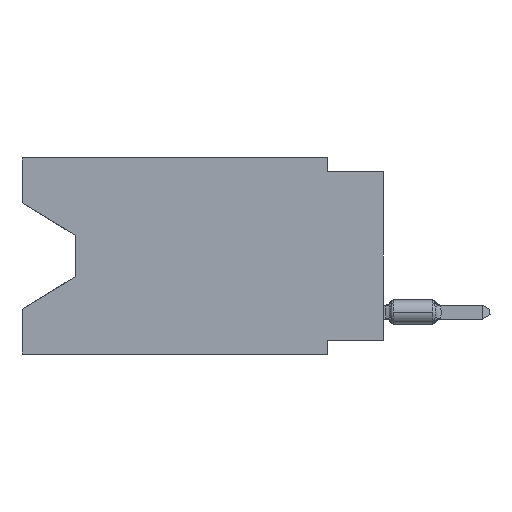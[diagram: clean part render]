
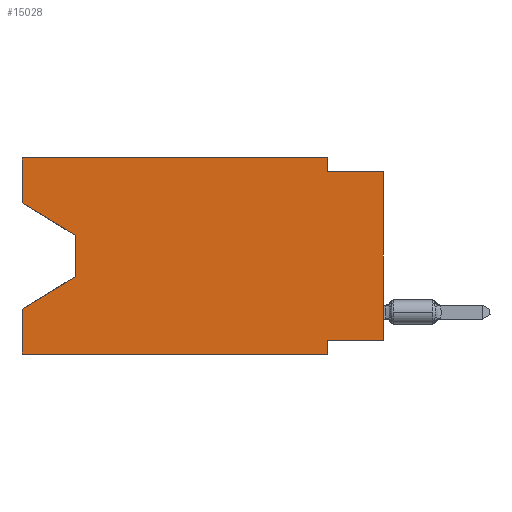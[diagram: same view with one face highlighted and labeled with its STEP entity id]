
A CAD part, left-side view. The second image highlights one B-rep face of the part: STEP entity #15028.
In plain terms, the highlighted planar face has unit normal (-1, 0, 0).
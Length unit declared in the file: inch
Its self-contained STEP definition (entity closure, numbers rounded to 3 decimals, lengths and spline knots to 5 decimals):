
#46 = CARTESIAN_POINT ( 'NONE',  ( 0., 0.645, 0. ) ) ;
#237 = DIRECTION ( 'NONE',  ( 1., 0., 0. ) ) ;
#358 = EDGE_CURVE ( 'NONE', #9131, #15385, #25712, .T. ) ;
#706 = CARTESIAN_POINT ( 'NONE',  ( 0., 0.645, 0. ) ) ;
#745 = VECTOR ( 'NONE', #42274, 39.37008 ) ;
#879 = CARTESIAN_POINT ( 'NONE',  ( 0., 0., -0.025 ) ) ;
#1329 = EDGE_LOOP ( 'NONE', ( #43893, #31554, #24257, #16277, #18783, #42385, #1953, #32774, #33896, #38609, #2377, #43063 ) ) ;
#1415 = DIRECTION ( 'NONE',  ( 0., -0.855, -0.519 ) ) ;
#1826 = VECTOR ( 'NONE', #4536, 39.37008 ) ;
#1953 = ORIENTED_EDGE ( 'NONE', *, *, #17842, .F. ) ;
#2377 = ORIENTED_EDGE ( 'NONE', *, *, #33016, .F. ) ;
#3323 = DIRECTION ( 'NONE',  ( 0., 0., -1. ) ) ;
#3434 = VERTEX_POINT ( 'NONE', #34422 ) ;
#3835 = CARTESIAN_POINT ( 'NONE',  ( 0., 0.645, -0.26975 ) ) ;
#4311 = LINE ( 'NONE', #879, #1826 ) ;
#4511 = VERTEX_POINT ( 'NONE', #46 ) ;
#4536 = DIRECTION ( 'NONE',  ( 0., -1., 0. ) ) ;
#5310 = LINE ( 'NONE', #26547, #37855 ) ;
#5850 = CARTESIAN_POINT ( 'NONE',  ( 0., 0.1, 0. ) ) ;
#7268 = VECTOR ( 'NONE', #38664, 39.37008 ) ;
#7551 = PLANE ( 'NONE',  #43920 ) ;
#8759 = VECTOR ( 'NONE', #3323, 39.37008 ) ;
#9131 = VERTEX_POINT ( 'NONE', #44432 ) ;
#9416 = VECTOR ( 'NONE', #21466, 39.37008 ) ;
#10140 = CARTESIAN_POINT ( 'NONE',  ( 0., 0., -0.025 ) ) ;
#10227 = CARTESIAN_POINT ( 'NONE',  ( 0., 0.1, -0.35 ) ) ;
#11408 = CARTESIAN_POINT ( 'NONE',  ( 0., 0.645, -0.35 ) ) ;
#11585 = CARTESIAN_POINT ( 'NONE',  ( 0., 0.55, -0.212 ) ) ;
#12826 = EDGE_CURVE ( 'NONE', #31599, #22382, #44892, .T. ) ;
#13238 = CARTESIAN_POINT ( 'NONE',  ( 0., 0.55, -0.138 ) ) ;
#14643 = LINE ( 'NONE', #706, #745 ) ;
#14780 = LINE ( 'NONE', #18657, #34609 ) ;
#14848 = CARTESIAN_POINT ( 'NONE',  ( 0., 0.645, 0. ) ) ;
#15028 = ADVANCED_FACE ( 'NONE', ( #18263 ), #7551, .F. ) ;
#15347 = VECTOR ( 'NONE', #32556, 39.37008 ) ;
#15385 = VERTEX_POINT ( 'NONE', #3835 ) ;
#16121 = DIRECTION ( 'NONE',  ( 0., 0., -1. ) ) ;
#16277 = ORIENTED_EDGE ( 'NONE', *, *, #358, .F. ) ;
#17458 = EDGE_CURVE ( 'NONE', #3434, #15385, #39215, .T. ) ;
#17842 = EDGE_CURVE ( 'NONE', #37685, #31599, #29112, .T. ) ;
#18263 = FACE_OUTER_BOUND ( 'NONE', #1329, .T. ) ;
#18418 = CARTESIAN_POINT ( 'NONE',  ( 0., 0.1, -0.325 ) ) ;
#18427 = DIRECTION ( 'NONE',  ( 0., -1., 0. ) ) ;
#18623 = CARTESIAN_POINT ( 'NONE',  ( 0., 0.645, 0. ) ) ;
#18657 = CARTESIAN_POINT ( 'NONE',  ( 0., 0.645, 0. ) ) ;
#18783 = ORIENTED_EDGE ( 'NONE', *, *, #40197, .T. ) ;
#19572 = CARTESIAN_POINT ( 'NONE',  ( 0., 0., 0. ) ) ;
#20453 = CARTESIAN_POINT ( 'NONE',  ( 0., 0.1, -0.35 ) ) ;
#21118 = VECTOR ( 'NONE', #39686, 39.37008 ) ;
#21466 = DIRECTION ( 'NONE',  ( 0., -1., 0. ) ) ;
#21486 = DIRECTION ( 'NONE',  ( 0., 0., -1. ) ) ;
#21542 = LINE ( 'NONE', #35683, #7268 ) ;
#22074 = EDGE_CURVE ( 'NONE', #45105, #25070, #4311, .T. ) ;
#22382 = VERTEX_POINT ( 'NONE', #10227 ) ;
#22799 = VECTOR ( 'NONE', #25983, 39.37008 ) ;
#23062 = VERTEX_POINT ( 'NONE', #37477 ) ;
#23440 = LINE ( 'NONE', #5850, #29016 ) ;
#23896 = EDGE_CURVE ( 'NONE', #23062, #45105, #23440, .T. ) ;
#24257 = ORIENTED_EDGE ( 'NONE', *, *, #17458, .T. ) ;
#25070 = VERTEX_POINT ( 'NONE', #10140 ) ;
#25178 = CARTESIAN_POINT ( 'NONE',  ( 0., 0., -0.325 ) ) ;
#25255 = CARTESIAN_POINT ( 'NONE',  ( 0., 0., -0.325 ) ) ;
#25367 = EDGE_CURVE ( 'NONE', #33323, #29673, #5310, .T. ) ;
#25712 = LINE ( 'NONE', #18623, #15347 ) ;
#25983 = DIRECTION ( 'NONE',  ( 0., 0.855, -0.519 ) ) ;
#26547 = CARTESIAN_POINT ( 'NONE',  ( 0., 0.645, -0.08025 ) ) ;
#26762 = EDGE_CURVE ( 'NONE', #33323, #4511, #14643, .T. ) ;
#27400 = EDGE_CURVE ( 'NONE', #37685, #25070, #33055, .T. ) ;
#27857 = EDGE_CURVE ( 'NONE', #29673, #3434, #21542, .T. ) ;
#28306 = LINE ( 'NONE', #11408, #9416 ) ;
#28832 = CARTESIAN_POINT ( 'NONE',  ( 0., 0.645, -0.08025 ) ) ;
#29016 = VECTOR ( 'NONE', #16121, 39.37008 ) ;
#29112 = LINE ( 'NONE', #25255, #30139 ) ;
#29673 = VERTEX_POINT ( 'NONE', #13238 ) ;
#30139 = VECTOR ( 'NONE', #42814, 39.37008 ) ;
#31554 = ORIENTED_EDGE ( 'NONE', *, *, #27857, .T. ) ;
#31570 = CARTESIAN_POINT ( 'NONE',  ( 0., 0.1, -0.025 ) ) ;
#31599 = VERTEX_POINT ( 'NONE', #18418 ) ;
#32556 = DIRECTION ( 'NONE',  ( 0., 0., 1. ) ) ;
#32774 = ORIENTED_EDGE ( 'NONE', *, *, #27400, .T. ) ;
#33016 = EDGE_CURVE ( 'NONE', #4511, #23062, #14780, .T. ) ;
#33055 = LINE ( 'NONE', #19572, #21118 ) ;
#33323 = VERTEX_POINT ( 'NONE', #28832 ) ;
#33896 = ORIENTED_EDGE ( 'NONE', *, *, #22074, .F. ) ;
#34422 = CARTESIAN_POINT ( 'NONE',  ( 0., 0.55, -0.212 ) ) ;
#34609 = VECTOR ( 'NONE', #18427, 39.37008 ) ;
#35683 = CARTESIAN_POINT ( 'NONE',  ( 0., 0.55, -0.138 ) ) ;
#37477 = CARTESIAN_POINT ( 'NONE',  ( 0., 0.1, 0. ) ) ;
#37685 = VERTEX_POINT ( 'NONE', #25178 ) ;
#37855 = VECTOR ( 'NONE', #1415, 39.37008 ) ;
#38609 = ORIENTED_EDGE ( 'NONE', *, *, #23896, .F. ) ;
#38664 = DIRECTION ( 'NONE',  ( 0., 0., -1. ) ) ;
#39215 = LINE ( 'NONE', #11585, #22799 ) ;
#39686 = DIRECTION ( 'NONE',  ( 0., 0., 1. ) ) ;
#40197 = EDGE_CURVE ( 'NONE', #9131, #22382, #28306, .T. ) ;
#42274 = DIRECTION ( 'NONE',  ( 0., 0., 1. ) ) ;
#42385 = ORIENTED_EDGE ( 'NONE', *, *, #12826, .F. ) ;
#42814 = DIRECTION ( 'NONE',  ( 0., 1., 0. ) ) ;
#43063 = ORIENTED_EDGE ( 'NONE', *, *, #26762, .F. ) ;
#43893 = ORIENTED_EDGE ( 'NONE', *, *, #25367, .T. ) ;
#43920 = AXIS2_PLACEMENT_3D ( 'NONE', #14848, #237, #21486 ) ;
#44432 = CARTESIAN_POINT ( 'NONE',  ( 0., 0.645, -0.35 ) ) ;
#44892 = LINE ( 'NONE', #20453, #8759 ) ;
#45105 = VERTEX_POINT ( 'NONE', #31570 ) ;
